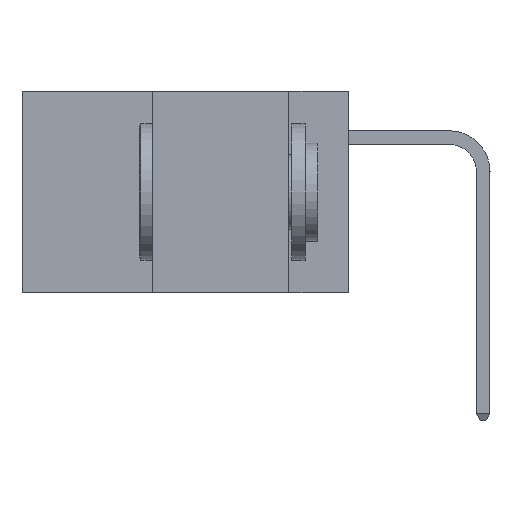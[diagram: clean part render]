
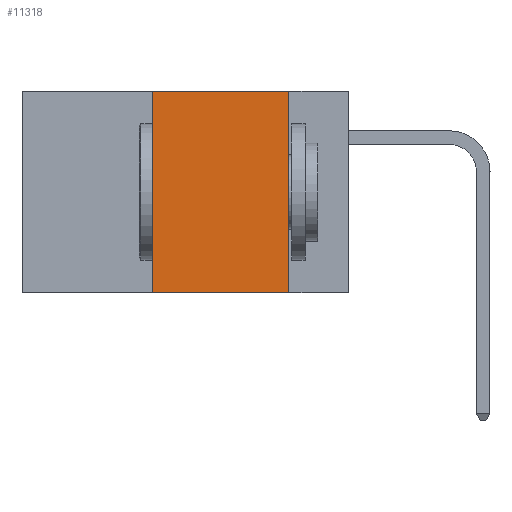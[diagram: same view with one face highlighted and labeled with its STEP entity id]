
A CAD part, left-side view. The second image highlights one B-rep face of the part: STEP entity #11318.
In plain terms, the highlighted planar face has unit normal (-1, 0, 0).
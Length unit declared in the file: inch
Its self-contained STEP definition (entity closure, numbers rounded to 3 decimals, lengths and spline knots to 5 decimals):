
#554 = CARTESIAN_POINT ( 'NONE',  ( 0., 0.11, 0. ) ) ;
#1561 = VECTOR ( 'NONE', #1582, 39.37008 ) ;
#1582 = DIRECTION ( 'NONE',  ( 0., -1., 0. ) ) ;
#2162 = VERTEX_POINT ( 'NONE', #9799 ) ;
#2328 = VECTOR ( 'NONE', #7366, 39.37008 ) ;
#2474 = ORIENTED_EDGE ( 'NONE', *, *, #11317, .T. ) ;
#3147 = AXIS2_PLACEMENT_3D ( 'NONE', #10192, #4639, #11138 ) ;
#3519 = CARTESIAN_POINT ( 'NONE',  ( 0., 0.6, 0. ) ) ;
#4035 = VERTEX_POINT ( 'NONE', #11944 ) ;
#4290 = VERTEX_POINT ( 'NONE', #10511 ) ;
#4420 = LINE ( 'NONE', #5506, #2328 ) ;
#4613 = DIRECTION ( 'NONE',  ( 0., 0., -1. ) ) ;
#4639 = DIRECTION ( 'NONE',  ( 1., 0., 0. ) ) ;
#5357 = VECTOR ( 'NONE', #10890, 39.37008 ) ;
#5506 = CARTESIAN_POINT ( 'NONE',  ( 0., 0.6, -0.37 ) ) ;
#6549 = EDGE_CURVE ( 'NONE', #4035, #7154, #11483, .T. ) ;
#7154 = VERTEX_POINT ( 'NONE', #554 ) ;
#7366 = DIRECTION ( 'NONE',  ( 0., -1., 0. ) ) ;
#7405 = PLANE ( 'NONE',  #3147 ) ;
#7624 = EDGE_CURVE ( 'NONE', #7154, #2162, #11021, .T. ) ;
#7898 = FACE_OUTER_BOUND ( 'NONE', #10637, .T. ) ;
#8964 = EDGE_CURVE ( 'NONE', #4290, #4035, #10124, .T. ) ;
#9383 = ORIENTED_EDGE ( 'NONE', *, *, #7624, .F. ) ;
#9704 = VECTOR ( 'NONE', #4613, 39.37008 ) ;
#9799 = CARTESIAN_POINT ( 'NONE',  ( 0., 0.11, -0.37 ) ) ;
#10124 = LINE ( 'NONE', #11867, #5357 ) ;
#10192 = CARTESIAN_POINT ( 'NONE',  ( 0., 0.6, 0. ) ) ;
#10511 = CARTESIAN_POINT ( 'NONE',  ( 0., 0.36, -0.37 ) ) ;
#10637 = EDGE_LOOP ( 'NONE', ( #9383, #10718, #11791, #2474 ) ) ;
#10718 = ORIENTED_EDGE ( 'NONE', *, *, #6549, .F. ) ;
#10890 = DIRECTION ( 'NONE',  ( 0., 0., 1. ) ) ;
#11021 = LINE ( 'NONE', #11961, #9704 ) ;
#11138 = DIRECTION ( 'NONE',  ( 0., 0., -1. ) ) ;
#11317 = EDGE_CURVE ( 'NONE', #4290, #2162, #4420, .T. ) ;
#11318 = ADVANCED_FACE ( 'NONE', ( #7898 ), #7405, .F. ) ;
#11483 = LINE ( 'NONE', #3519, #1561 ) ;
#11791 = ORIENTED_EDGE ( 'NONE', *, *, #8964, .F. ) ;
#11867 = CARTESIAN_POINT ( 'NONE',  ( 0., 0.36, 0. ) ) ;
#11944 = CARTESIAN_POINT ( 'NONE',  ( 0., 0.36, 0. ) ) ;
#11961 = CARTESIAN_POINT ( 'NONE',  ( 0., 0.11, 0. ) ) ;
